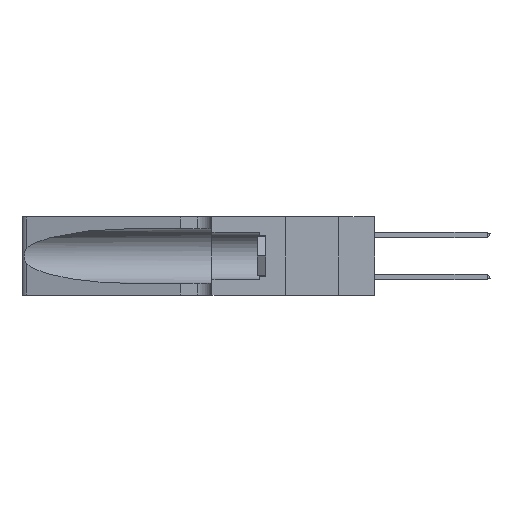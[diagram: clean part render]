
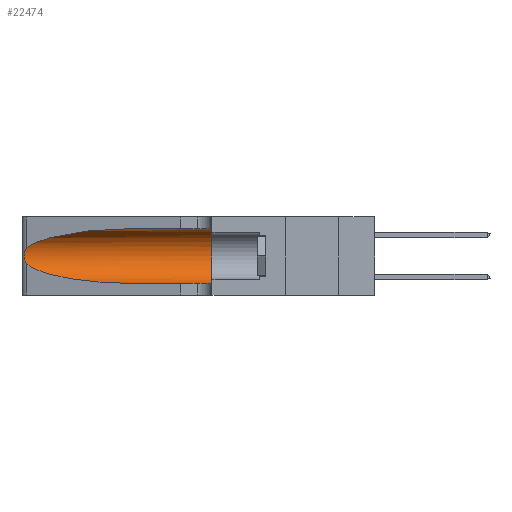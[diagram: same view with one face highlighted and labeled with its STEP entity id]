
A CAD part, left-side view. The second image highlights one B-rep face of the part: STEP entity #22474.
In plain terms, the highlighted cylindrical face has radius 3.308 mm (diameter 6.617 mm), a partial arc.
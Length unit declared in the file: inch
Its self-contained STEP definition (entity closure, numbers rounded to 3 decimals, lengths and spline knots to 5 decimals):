
#726 = CYLINDRICAL_SURFACE ( 'NONE', #8640, 0.13025 ) ;
#853 = CARTESIAN_POINT ( 'NONE',  ( 0.25856, 1.23593, 0.16098 ) ) ;
#1719 = FACE_OUTER_BOUND ( 'NONE', #37669, .T. ) ;
#2387 = DIRECTION ( 'NONE',  ( 0., 1., 0. ) ) ;
#2849 = DIRECTION ( 'NONE',  ( 0., 0., -1. ) ) ;
#3029 = VECTOR ( 'NONE', #15642, 39.37008 ) ;
#3284 =( BOUNDED_CURVE ( )  B_SPLINE_CURVE ( 3, ( #33004, #17661, #17799, #39114 ),
 .UNSPECIFIED., .F., .T. ) 
 B_SPLINE_CURVE_WITH_KNOTS ( ( 4, 4 ),
 ( 1.5708, 2.84003 ),
 .UNSPECIFIED. ) 
 CURVE ( )  GEOMETRIC_REPRESENTATION_ITEM ( )  RATIONAL_B_SPLINE_CURVE ( ( 1., 0.87, 0.87, 1. ) ) 
 REPRESENTATION_ITEM ( '' )  );
#3552 = ORIENTED_EDGE ( 'NONE', *, *, #16148, .F. ) ;
#4043 = CARTESIAN_POINT ( 'NONE',  ( 0.25639, 1.23186, 0.15144 ) ) ;
#4841 = VERTEX_POINT ( 'NONE', #14696 ) ;
#5247 = CARTESIAN_POINT ( 'NONE',  ( 0.2373, 1.15595, 0.08982 ) ) ;
#7207 = CARTESIAN_POINT ( 'NONE',  ( 0.25487, 1.22718, 0.14631 ) ) ;
#7573 = AXIS2_PLACEMENT_3D ( 'NONE', #20935, #2387, #23985 ) ;
#8640 = AXIS2_PLACEMENT_3D ( 'NONE', #15402, #33644, #2849 ) ;
#10186 = CARTESIAN_POINT ( 'NONE',  ( 0.25639, 1.23184, 0.21858 ) ) ;
#13280 = CARTESIAN_POINT ( 'NONE',  ( 0.25854, 1.2359, 0.20912 ) ) ;
#13543 =( BOUNDED_CURVE ( )  B_SPLINE_CURVE ( 3, ( #23639, #5247, #32871, #14594 ),
 .UNSPECIFIED., .F., .T. ) 
 B_SPLINE_CURVE_WITH_KNOTS ( ( 4, 4 ),
 ( 3.44316, 4.71239 ),
 .UNSPECIFIED. ) 
 CURVE ( )  GEOMETRIC_REPRESENTATION_ITEM ( )  RATIONAL_B_SPLINE_CURVE ( ( 1., 0.87, 0.87, 1. ) ) 
 REPRESENTATION_ITEM ( '' )  );
#13907 = VERTEX_POINT ( 'NONE', #18042 ) ;
#14594 = CARTESIAN_POINT ( 'NONE',  ( 0.1305, 0.72297, 0.05475 ) ) ;
#14696 = CARTESIAN_POINT ( 'NONE',  ( 0.1305, 0.35, 0.05475 ) ) ;
#15205 = CARTESIAN_POINT ( 'NONE',  ( 0.1305, 0.35, 0.31525 ) ) ;
#15392 = CARTESIAN_POINT ( 'NONE',  ( 0.1305, 0.72297, 0.31525 ) ) ;
#15402 = CARTESIAN_POINT ( 'NONE',  ( 0.1305, 1.61858, 0.185 ) ) ;
#15642 = DIRECTION ( 'NONE',  ( 0., -1., 0. ) ) ;
#15830 = CARTESIAN_POINT ( 'NONE',  ( 0.1305, 0.72297, 0.05475 ) ) ;
#16148 = EDGE_CURVE ( 'NONE', #20613, #23349, #20491, .T. ) ;
#16269 = CARTESIAN_POINT ( 'NONE',  ( 0.25555, 1.22994, 0.2215 ) ) ;
#16412 = CARTESIAN_POINT ( 'NONE',  ( 0.26075, 1.23896, 0.19203 ) ) ;
#16454 = DIRECTION ( 'NONE',  ( 0., -1., 0. ) ) ;
#17569 = VERTEX_POINT ( 'NONE', #23735 ) ;
#17661 = CARTESIAN_POINT ( 'NONE',  ( 0.18966, 0.96281, 0.31525 ) ) ;
#17799 = CARTESIAN_POINT ( 'NONE',  ( 0.2373, 1.15595, 0.28018 ) ) ;
#18042 = CARTESIAN_POINT ( 'NONE',  ( 0.25487, 1.22718, 0.14631 ) ) ;
#18474 = ORIENTED_EDGE ( 'NONE', *, *, #29092, .T. ) ;
#18840 = ORIENTED_EDGE ( 'NONE', *, *, #32812, .T. ) ;
#19457 = CARTESIAN_POINT ( 'NONE',  ( 0.26017, 1.23833, 0.17102 ) ) ;
#19503 = CARTESIAN_POINT ( 'NONE',  ( 0.1305, 1.61858, 0.05475 ) ) ;
#20491 = LINE ( 'NONE', #29012, #3029 ) ;
#20608 = ORIENTED_EDGE ( 'NONE', *, *, #26748, .T. ) ;
#20613 = VERTEX_POINT ( 'NONE', #15392 ) ;
#20663 = B_SPLINE_CURVE_WITH_KNOTS ( 'NONE', 3,
 ( #22357, #16269, #10186, #31590, #13280, #34637, #16412, #37716, #19457, #853, #22493, #4043, #25548, #7207 ),
 .UNSPECIFIED., .F., .F.,
 ( 4, 2, 2, 2, 2, 2, 4 ),
 ( 0., 0.00027, 0.00053, 0.00107, 0.0016, 0.00187, 0.00214 ),
 .UNSPECIFIED. ) ;
#20935 = CARTESIAN_POINT ( 'NONE',  ( 0.1305, 0.35, 0.185 ) ) ;
#21161 = EDGE_CURVE ( 'NONE', #23349, #4841, #34558, .T. ) ;
#22045 = VERTEX_POINT ( 'NONE', #15830 ) ;
#22357 = CARTESIAN_POINT ( 'NONE',  ( 0.25487, 1.22718, 0.22369 ) ) ;
#22474 = ADVANCED_FACE ( 'NONE', ( #1719 ), #726, .F. ) ;
#22493 = CARTESIAN_POINT ( 'NONE',  ( 0.25789, 1.23486, 0.15765 ) ) ;
#23349 = VERTEX_POINT ( 'NONE', #15205 ) ;
#23639 = CARTESIAN_POINT ( 'NONE',  ( 0.25487, 1.22718, 0.14631 ) ) ;
#23735 = CARTESIAN_POINT ( 'NONE',  ( 0.25487, 1.22718, 0.22369 ) ) ;
#23985 = DIRECTION ( 'NONE',  ( 0., 0., 1. ) ) ;
#25548 = CARTESIAN_POINT ( 'NONE',  ( 0.25555, 1.22993, 0.14849 ) ) ;
#26748 = EDGE_CURVE ( 'NONE', #20613, #17569, #3284, .T. ) ;
#29012 = CARTESIAN_POINT ( 'NONE',  ( 0.1305, 1.61858, 0.31525 ) ) ;
#29092 = EDGE_CURVE ( 'NONE', #22045, #4841, #38497, .T. ) ;
#30371 = VECTOR ( 'NONE', #16454, 39.37008 ) ;
#31590 = CARTESIAN_POINT ( 'NONE',  ( 0.25787, 1.23484, 0.2124 ) ) ;
#32812 = EDGE_CURVE ( 'NONE', #13907, #22045, #13543, .T. ) ;
#32871 = CARTESIAN_POINT ( 'NONE',  ( 0.18966, 0.96281, 0.05475 ) ) ;
#33004 = CARTESIAN_POINT ( 'NONE',  ( 0.1305, 0.72297, 0.31525 ) ) ;
#33222 = ORIENTED_EDGE ( 'NONE', *, *, #21161, .F. ) ;
#33363 = ORIENTED_EDGE ( 'NONE', *, *, #33892, .T. ) ;
#33644 = DIRECTION ( 'NONE',  ( 0., -1., 0. ) ) ;
#33892 = EDGE_CURVE ( 'NONE', #17569, #13907, #20663, .T. ) ;
#34558 = CIRCLE ( 'NONE', #7573, 0.13025 ) ;
#34637 = CARTESIAN_POINT ( 'NONE',  ( 0.26018, 1.23835, 0.19895 ) ) ;
#37669 = EDGE_LOOP ( 'NONE', ( #20608, #33363, #18840, #18474, #33222, #3552 ) ) ;
#37716 = CARTESIAN_POINT ( 'NONE',  ( 0.26075, 1.23896, 0.178 ) ) ;
#38497 = LINE ( 'NONE', #19503, #30371 ) ;
#39114 = CARTESIAN_POINT ( 'NONE',  ( 0.25487, 1.22718, 0.22369 ) ) ;
